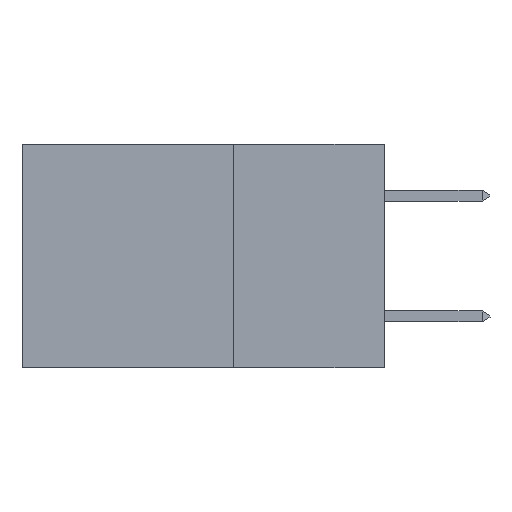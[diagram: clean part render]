
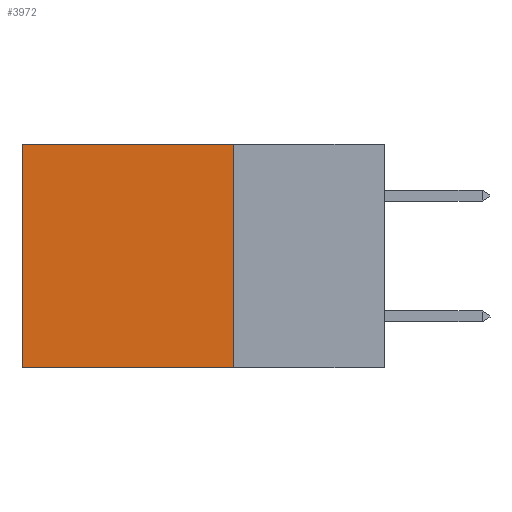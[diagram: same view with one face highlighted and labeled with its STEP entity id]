
A CAD part, left-side view. The second image highlights one B-rep face of the part: STEP entity #3972.
In plain terms, the highlighted planar face has unit normal (-1, 0, 0).
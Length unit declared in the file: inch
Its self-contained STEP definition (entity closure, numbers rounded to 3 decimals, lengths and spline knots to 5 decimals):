
#288 = CARTESIAN_POINT ( 'NONE',  ( 0.2875, 0.6, 0. ) ) ;
#1817 = VECTOR ( 'NONE', #20151, 39.37008 ) ;
#2105 = VERTEX_POINT ( 'NONE', #16742 ) ;
#2138 = PLANE ( 'NONE',  #19731 ) ;
#2251 = CARTESIAN_POINT ( 'NONE',  ( 0.2875, 0.25, 0. ) ) ;
#3972 = ADVANCED_FACE ( 'NONE', ( #10860 ), #2138, .F. ) ;
#5297 = EDGE_CURVE ( 'NONE', #13757, #2105, #8085, .T. ) ;
#5427 = CARTESIAN_POINT ( 'NONE',  ( 0.2875, 0.6, -0.37 ) ) ;
#5787 = CARTESIAN_POINT ( 'NONE',  ( 0.2875, 0.25, 0. ) ) ;
#5878 = CARTESIAN_POINT ( 'NONE',  ( 0.2875, 0.25, -0.37 ) ) ;
#5957 = DIRECTION ( 'NONE',  ( 0., 1., 0. ) ) ;
#6280 = VERTEX_POINT ( 'NONE', #5427 ) ;
#6282 = DIRECTION ( 'NONE',  ( 0., 0., -1. ) ) ;
#8085 = LINE ( 'NONE', #11515, #17017 ) ;
#8302 = EDGE_CURVE ( 'NONE', #13757, #19715, #11317, .T. ) ;
#9252 = LINE ( 'NONE', #5878, #22750 ) ;
#9369 = DIRECTION ( 'NONE',  ( 1., 0., 0. ) ) ;
#10270 = LINE ( 'NONE', #288, #19808 ) ;
#10860 = FACE_OUTER_BOUND ( 'NONE', #16639, .T. ) ;
#11317 = LINE ( 'NONE', #2251, #1817 ) ;
#11515 = CARTESIAN_POINT ( 'NONE',  ( 0.2875, 0.25, 0. ) ) ;
#13322 = ORIENTED_EDGE ( 'NONE', *, *, #19955, .T. ) ;
#13599 = EDGE_CURVE ( 'NONE', #2105, #6280, #9252, .T. ) ;
#13757 = VERTEX_POINT ( 'NONE', #22262 ) ;
#16639 = EDGE_LOOP ( 'NONE', ( #13322, #21460, #18360, #17589 ) ) ;
#16742 = CARTESIAN_POINT ( 'NONE',  ( 0.2875, 0.25, -0.37 ) ) ;
#17017 = VECTOR ( 'NONE', #6282, 39.37008 ) ;
#17589 = ORIENTED_EDGE ( 'NONE', *, *, #8302, .T. ) ;
#18280 = DIRECTION ( 'NONE',  ( 0., 0., -1. ) ) ;
#18360 = ORIENTED_EDGE ( 'NONE', *, *, #5297, .F. ) ;
#19715 = VERTEX_POINT ( 'NONE', #21148 ) ;
#19731 = AXIS2_PLACEMENT_3D ( 'NONE', #5787, #9369, #21754 ) ;
#19808 = VECTOR ( 'NONE', #18280, 39.37008 ) ;
#19955 = EDGE_CURVE ( 'NONE', #19715, #6280, #10270, .T. ) ;
#20151 = DIRECTION ( 'NONE',  ( 0., 1., 0. ) ) ;
#21148 = CARTESIAN_POINT ( 'NONE',  ( 0.2875, 0.6, 0. ) ) ;
#21460 = ORIENTED_EDGE ( 'NONE', *, *, #13599, .F. ) ;
#21754 = DIRECTION ( 'NONE',  ( 0., 0., -1. ) ) ;
#22262 = CARTESIAN_POINT ( 'NONE',  ( 0.2875, 0.25, 0. ) ) ;
#22750 = VECTOR ( 'NONE', #5957, 39.37008 ) ;
